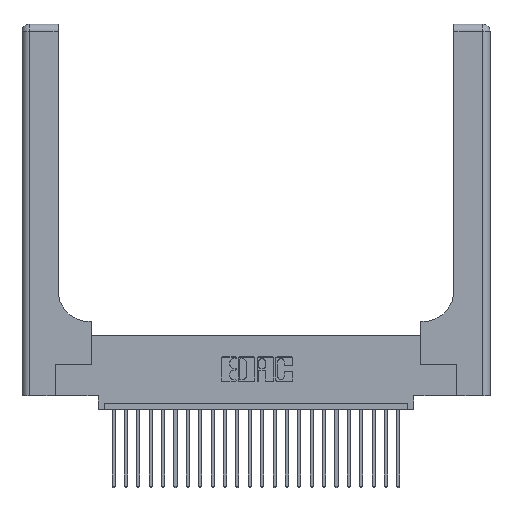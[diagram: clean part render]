
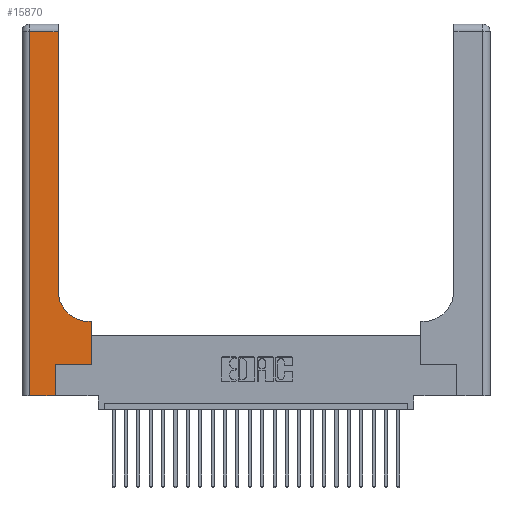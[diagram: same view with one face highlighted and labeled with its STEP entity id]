
A CAD part, top view. The second image highlights one B-rep face of the part: STEP entity #15870.
In plain terms, the highlighted planar face has unit normal (0, 0, 1).
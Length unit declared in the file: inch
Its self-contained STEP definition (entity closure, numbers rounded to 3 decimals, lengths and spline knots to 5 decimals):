
#86 = DIRECTION ( 'NONE',  ( 0., 1., 0. ) ) ;
#581 = ORIENTED_EDGE ( 'NONE', *, *, #5576, .T. ) ;
#967 = DIRECTION ( 'NONE',  ( -1., 0., 0. ) ) ;
#980 = ORIENTED_EDGE ( 'NONE', *, *, #2455, .T. ) ;
#1121 = CARTESIAN_POINT ( 'NONE',  ( 0.269, 0.25, 0.37 ) ) ;
#1273 = CARTESIAN_POINT ( 'NONE',  ( 0.269, 0., 0.37 ) ) ;
#1500 = CARTESIAN_POINT ( 'NONE',  ( 0.5585, 0.6, 0.37 ) ) ;
#2455 = EDGE_CURVE ( 'NONE', #15390, #12970, #19936, .T. ) ;
#2638 = VERTEX_POINT ( 'NONE', #12321 ) ;
#3025 = PLANE ( 'NONE',  #7888 ) ;
#3358 = EDGE_CURVE ( 'NONE', #6459, #22191, #10841, .T. ) ;
#3384 = DIRECTION ( 'NONE',  ( -1., 0., 0. ) ) ;
#3788 = EDGE_CURVE ( 'NONE', #22191, #19200, #22656, .T. ) ;
#4094 = CARTESIAN_POINT ( 'NONE',  ( 0.2915, 0.85, 0.37 ) ) ;
#4096 = VERTEX_POINT ( 'NONE', #20120 ) ;
#4297 = CARTESIAN_POINT ( 'NONE',  ( 0.5415, 0.85, 0.37 ) ) ;
#4456 = VERTEX_POINT ( 'NONE', #4094 ) ;
#5576 = EDGE_CURVE ( 'NONE', #12970, #6459, #11971, .T. ) ;
#5681 = DIRECTION ( 'NONE',  ( 0., 1., 0. ) ) ;
#6360 = LINE ( 'NONE', #6826, #17578 ) ;
#6459 = VERTEX_POINT ( 'NONE', #19895 ) ;
#6826 = CARTESIAN_POINT ( 'NONE',  ( 0., 2.94, 0.37 ) ) ;
#7185 = ORIENTED_EDGE ( 'NONE', *, *, #14847, .T. ) ;
#7599 = CARTESIAN_POINT ( 'NONE',  ( 0.2915, 3., 0.37 ) ) ;
#7850 = FACE_OUTER_BOUND ( 'NONE', #10658, .T. ) ;
#7888 = AXIS2_PLACEMENT_3D ( 'NONE', #19148, #25211, #3384 ) ;
#8332 = EDGE_CURVE ( 'NONE', #4456, #2638, #22631, .T. ) ;
#9106 = VECTOR ( 'NONE', #16158, 39.37008 ) ;
#9670 = ORIENTED_EDGE ( 'NONE', *, *, #24138, .T. ) ;
#10008 = LINE ( 'NONE', #16069, #9106 ) ;
#10658 = EDGE_LOOP ( 'NONE', ( #16616, #7185, #17947, #980, #581, #14851, #17933, #18511, #9670 ) ) ;
#10841 = LINE ( 'NONE', #1121, #23910 ) ;
#10847 = CARTESIAN_POINT ( 'NONE',  ( 0.269, 0., 0.37 ) ) ;
#11971 = LINE ( 'NONE', #10847, #15110 ) ;
#12001 = VERTEX_POINT ( 'NONE', #22888 ) ;
#12321 = CARTESIAN_POINT ( 'NONE',  ( 0.2915, 2.94, 0.37 ) ) ;
#12970 = VERTEX_POINT ( 'NONE', #1273 ) ;
#13390 = VECTOR ( 'NONE', #20523, 39.37008 ) ;
#13406 = CIRCLE ( 'NONE', #21528, 0.25 ) ;
#13620 = CARTESIAN_POINT ( 'NONE',  ( 0.5585, 0.25, 0.37 ) ) ;
#13691 = EDGE_CURVE ( 'NONE', #4096, #15390, #21038, .T. ) ;
#14234 = VECTOR ( 'NONE', #5681, 39.37008 ) ;
#14447 = CARTESIAN_POINT ( 'NONE',  ( 0., 0., 0.37 ) ) ;
#14612 = DIRECTION ( 'NONE',  ( 0., 1., 0. ) ) ;
#14847 = EDGE_CURVE ( 'NONE', #2638, #4096, #6360, .T. ) ;
#14851 = ORIENTED_EDGE ( 'NONE', *, *, #3358, .T. ) ;
#15110 = VECTOR ( 'NONE', #14612, 39.37008 ) ;
#15390 = VERTEX_POINT ( 'NONE', #15844 ) ;
#15496 = DIRECTION ( 'NONE',  ( 1., 0., 0. ) ) ;
#15844 = CARTESIAN_POINT ( 'NONE',  ( 0.06, 0., 0.37 ) ) ;
#15870 = ADVANCED_FACE ( 'NONE', ( #7850 ), #3025, .F. ) ;
#16069 = CARTESIAN_POINT ( 'NONE',  ( 0.2915, 0.6, 0.37 ) ) ;
#16135 = DIRECTION ( 'NONE',  ( 1., 0., 0. ) ) ;
#16158 = DIRECTION ( 'NONE',  ( -1., 0., 0. ) ) ;
#16205 = CARTESIAN_POINT ( 'NONE',  ( 0.5585, 0.25, 0.37 ) ) ;
#16616 = ORIENTED_EDGE ( 'NONE', *, *, #8332, .T. ) ;
#17578 = VECTOR ( 'NONE', #967, 39.37008 ) ;
#17933 = ORIENTED_EDGE ( 'NONE', *, *, #3788, .T. ) ;
#17947 = ORIENTED_EDGE ( 'NONE', *, *, #13691, .T. ) ;
#18238 = DIRECTION ( 'NONE',  ( 0., 0., -1. ) ) ;
#18511 = ORIENTED_EDGE ( 'NONE', *, *, #23564, .T. ) ;
#19148 = CARTESIAN_POINT ( 'NONE',  ( 0., 3., 0.37 ) ) ;
#19200 = VERTEX_POINT ( 'NONE', #1500 ) ;
#19895 = CARTESIAN_POINT ( 'NONE',  ( 0.269, 0.25, 0.37 ) ) ;
#19936 = LINE ( 'NONE', #14447, #13390 ) ;
#20120 = CARTESIAN_POINT ( 'NONE',  ( 0.06, 2.94, 0.37 ) ) ;
#20523 = DIRECTION ( 'NONE',  ( 1., 0., 0. ) ) ;
#21038 = LINE ( 'NONE', #22926, #24752 ) ;
#21528 = AXIS2_PLACEMENT_3D ( 'NONE', #4297, #18238, #16135 ) ;
#22191 = VERTEX_POINT ( 'NONE', #13620 ) ;
#22631 = LINE ( 'NONE', #7599, #14234 ) ;
#22656 = LINE ( 'NONE', #16205, #25781 ) ;
#22888 = CARTESIAN_POINT ( 'NONE',  ( 0.5415, 0.6, 0.37 ) ) ;
#22926 = CARTESIAN_POINT ( 'NONE',  ( 0.06, 3., 0.37 ) ) ;
#23564 = EDGE_CURVE ( 'NONE', #19200, #12001, #10008, .T. ) ;
#23910 = VECTOR ( 'NONE', #15496, 39.37008 ) ;
#23947 = DIRECTION ( 'NONE',  ( 0., -1., 0. ) ) ;
#24138 = EDGE_CURVE ( 'NONE', #12001, #4456, #13406, .T. ) ;
#24752 = VECTOR ( 'NONE', #23947, 39.37008 ) ;
#25211 = DIRECTION ( 'NONE',  ( 0., 0., -1. ) ) ;
#25781 = VECTOR ( 'NONE', #86, 39.37008 ) ;
